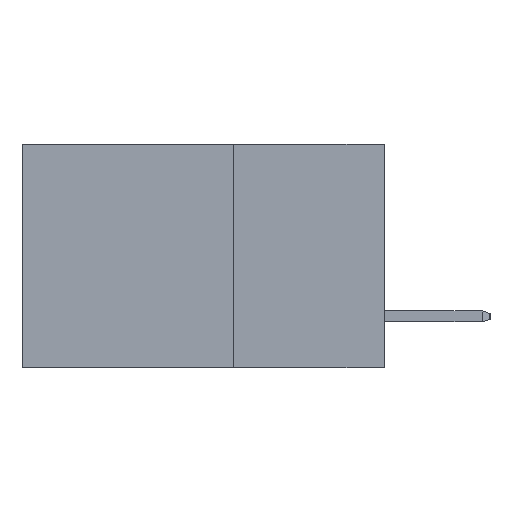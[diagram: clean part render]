
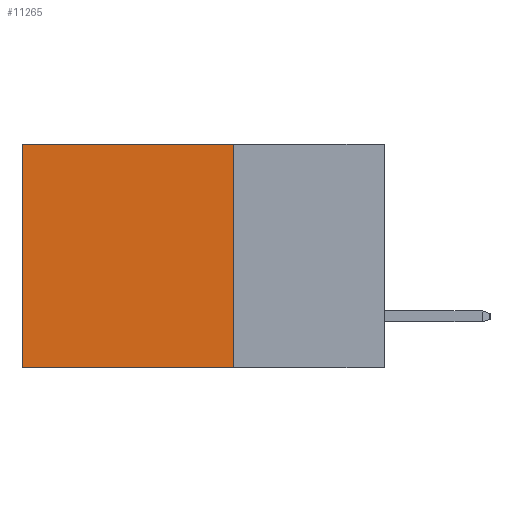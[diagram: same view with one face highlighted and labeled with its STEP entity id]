
A CAD part, left-side view. The second image highlights one B-rep face of the part: STEP entity #11265.
In plain terms, the highlighted planar face has unit normal (-1, 0, 0).
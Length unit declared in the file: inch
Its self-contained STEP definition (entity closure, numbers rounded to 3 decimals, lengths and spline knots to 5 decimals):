
#78 = AXIS2_PLACEMENT_3D ( 'NONE', #5528, #16567, #7116 ) ;
#901 = VERTEX_POINT ( 'NONE', #15079 ) ;
#1065 = VECTOR ( 'NONE', #10321, 39.37008 ) ;
#2527 = VECTOR ( 'NONE', #11612, 39.37008 ) ;
#2849 = VERTEX_POINT ( 'NONE', #13050 ) ;
#3165 = VERTEX_POINT ( 'NONE', #5042 ) ;
#3996 = LINE ( 'NONE', #19096, #4946 ) ;
#4024 = PLANE ( 'NONE',  #78 ) ;
#4056 = VECTOR ( 'NONE', #11186, 39.37008 ) ;
#4682 = VERTEX_POINT ( 'NONE', #7636 ) ;
#4946 = VECTOR ( 'NONE', #8105, 39.37008 ) ;
#5042 = CARTESIAN_POINT ( 'NONE',  ( 0.2615, 0.6, -0.37 ) ) ;
#5347 = EDGE_CURVE ( 'NONE', #901, #3165, #8203, .T. ) ;
#5528 = CARTESIAN_POINT ( 'NONE',  ( 0.2615, 0.25, -0.37 ) ) ;
#5870 = ORIENTED_EDGE ( 'NONE', *, *, #9929, .F. ) ;
#7116 = DIRECTION ( 'NONE',  ( 0., 0., -1. ) ) ;
#7636 = CARTESIAN_POINT ( 'NONE',  ( 0.2615, 0.25, 0. ) ) ;
#8105 = DIRECTION ( 'NONE',  ( 0., 0., -1. ) ) ;
#8203 = LINE ( 'NONE', #11233, #4056 ) ;
#8486 = ORIENTED_EDGE ( 'NONE', *, *, #5347, .F. ) ;
#8755 = CARTESIAN_POINT ( 'NONE',  ( 0.2615, 0.25, -0.37 ) ) ;
#9388 = LINE ( 'NONE', #8755, #1065 ) ;
#9929 = EDGE_CURVE ( 'NONE', #4682, #901, #9388, .T. ) ;
#10321 = DIRECTION ( 'NONE',  ( 0., 0., -1. ) ) ;
#10810 = LINE ( 'NONE', #19374, #2527 ) ;
#11074 = EDGE_CURVE ( 'NONE', #2849, #3165, #3996, .T. ) ;
#11186 = DIRECTION ( 'NONE',  ( 0., 1., 0. ) ) ;
#11233 = CARTESIAN_POINT ( 'NONE',  ( 0.2615, 0.25, -0.37 ) ) ;
#11265 = ADVANCED_FACE ( 'NONE', ( #12025 ), #4024, .F. ) ;
#11612 = DIRECTION ( 'NONE',  ( 0., 1., 0. ) ) ;
#12025 = FACE_OUTER_BOUND ( 'NONE', #15554, .T. ) ;
#13050 = CARTESIAN_POINT ( 'NONE',  ( 0.2615, 0.6, 0. ) ) ;
#15079 = CARTESIAN_POINT ( 'NONE',  ( 0.2615, 0.25, -0.37 ) ) ;
#15343 = EDGE_CURVE ( 'NONE', #4682, #2849, #10810, .T. ) ;
#15554 = EDGE_LOOP ( 'NONE', ( #18707, #8486, #5870, #20153 ) ) ;
#16567 = DIRECTION ( 'NONE',  ( 1., 0., 0. ) ) ;
#18707 = ORIENTED_EDGE ( 'NONE', *, *, #11074, .T. ) ;
#19096 = CARTESIAN_POINT ( 'NONE',  ( 0.2615, 0.6, -0.37 ) ) ;
#19374 = CARTESIAN_POINT ( 'NONE',  ( 0.2615, 0.25, 0. ) ) ;
#20153 = ORIENTED_EDGE ( 'NONE', *, *, #15343, .T. ) ;
